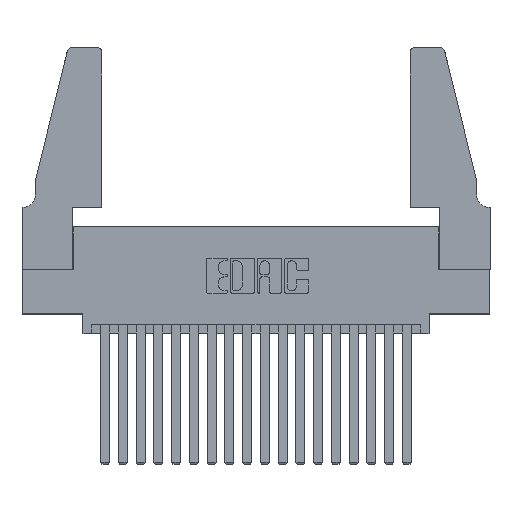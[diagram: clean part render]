
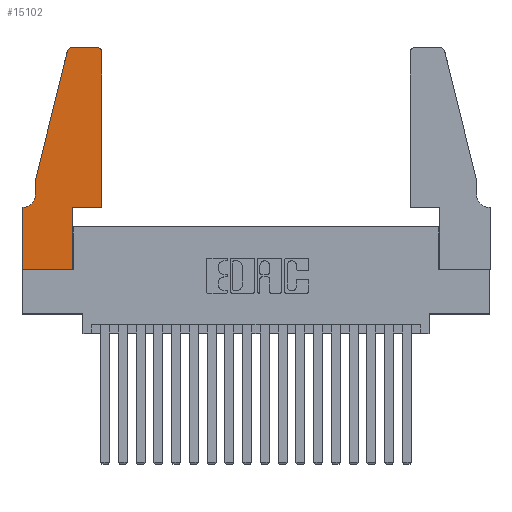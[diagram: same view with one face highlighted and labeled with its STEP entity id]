
A CAD part, top view. The second image highlights one B-rep face of the part: STEP entity #15102.
In plain terms, the highlighted planar face has unit normal (0, 0, 1).
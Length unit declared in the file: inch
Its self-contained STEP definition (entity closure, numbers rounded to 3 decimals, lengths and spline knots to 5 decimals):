
#88 = DIRECTION ( 'NONE',  ( 1., 0., 0. ) ) ;
#147 = DIRECTION ( 'NONE',  ( 0., 1., 0. ) ) ;
#178 = LINE ( 'NONE', #14275, #7966 ) ;
#248 = CARTESIAN_POINT ( 'NONE',  ( 0., 0.35, 0.37 ) ) ;
#522 = ORIENTED_EDGE ( 'NONE', *, *, #8987, .T. ) ;
#708 = CARTESIAN_POINT ( 'NONE',  ( 0.0755, 0.35, 0.37 ) ) ;
#824 = CARTESIAN_POINT ( 'NONE',  ( 0.2865, 0., 0.37 ) ) ;
#938 = VECTOR ( 'NONE', #147, 39.37008 ) ;
#967 = EDGE_LOOP ( 'NONE', ( #17690, #7799, #4221, #8732, #2994, #7582, #4954, #1731, #14276, #15666, #522, #7607 ) ) ;
#1402 = LINE ( 'NONE', #3292, #938 ) ;
#1456 = EDGE_CURVE ( 'NONE', #5873, #14737, #15552, .T. ) ;
#1731 = ORIENTED_EDGE ( 'NONE', *, *, #8331, .T. ) ;
#1837 = PLANE ( 'NONE',  #11635 ) ;
#2092 = VECTOR ( 'NONE', #7995, 39.37008 ) ;
#2198 = CARTESIAN_POINT ( 'NONE',  ( 0.4505, 0.35, 0.37 ) ) ;
#2199 = VERTEX_POINT ( 'NONE', #11678 ) ;
#2308 = VERTEX_POINT ( 'NONE', #9974 ) ;
#2362 = DIRECTION ( 'NONE',  ( 0., 1., 0. ) ) ;
#2425 = EDGE_CURVE ( 'NONE', #12426, #5873, #17566, .T. ) ;
#2835 = AXIS2_PLACEMENT_3D ( 'NONE', #18126, #9344, #88 ) ;
#2994 = ORIENTED_EDGE ( 'NONE', *, *, #18997, .T. ) ;
#3292 = CARTESIAN_POINT ( 'NONE',  ( 0.2865, 0.35, 0.37 ) ) ;
#3478 = DIRECTION ( 'NONE',  ( 0., 0., 1. ) ) ;
#3642 = VECTOR ( 'NONE', #13840, 39.37008 ) ;
#3739 = AXIS2_PLACEMENT_3D ( 'NONE', #7077, #17346, #8544 ) ;
#3792 = LINE ( 'NONE', #2198, #14749 ) ;
#3895 = DIRECTION ( 'NONE',  ( -1., 0., 0. ) ) ;
#3970 = CARTESIAN_POINT ( 'NONE',  ( 0., 0., 0.37 ) ) ;
#4125 = CARTESIAN_POINT ( 'NONE',  ( 0.25487, 1.22718, 0.37 ) ) ;
#4221 = ORIENTED_EDGE ( 'NONE', *, *, #2425, .T. ) ;
#4752 = VERTEX_POINT ( 'NONE', #10241 ) ;
#4954 = ORIENTED_EDGE ( 'NONE', *, *, #5242, .T. ) ;
#5242 = EDGE_CURVE ( 'NONE', #16561, #13067, #178, .T. ) ;
#5262 = EDGE_CURVE ( 'NONE', #18013, #16561, #15336, .T. ) ;
#5575 = CIRCLE ( 'NONE', #3739, 0.03 ) ;
#5873 = VERTEX_POINT ( 'NONE', #11477 ) ;
#5892 = VERTEX_POINT ( 'NONE', #824 ) ;
#6156 = EDGE_CURVE ( 'NONE', #5892, #2308, #1402, .T. ) ;
#6616 = CARTESIAN_POINT ( 'NONE',  ( 0.0055, 0.42, 0.37 ) ) ;
#7077 = CARTESIAN_POINT ( 'NONE',  ( 0.284, 1.22, 0.37 ) ) ;
#7582 = ORIENTED_EDGE ( 'NONE', *, *, #5262, .T. ) ;
#7607 = ORIENTED_EDGE ( 'NONE', *, *, #18281, .T. ) ;
#7799 = ORIENTED_EDGE ( 'NONE', *, *, #16663, .T. ) ;
#7966 = VECTOR ( 'NONE', #8418, 39.37008 ) ;
#7995 = DIRECTION ( 'NONE',  ( -0.239, -0.971, 0. ) ) ;
#8025 = CARTESIAN_POINT ( 'NONE',  ( 0.0755, 0.5, 0.37 ) ) ;
#8038 = CIRCLE ( 'NONE', #18081, 0.07 ) ;
#8085 = DIRECTION ( 'NONE',  ( -1., 0., 0. ) ) ;
#8144 = CARTESIAN_POINT ( 'NONE',  ( 0.2605, 1.25, 0.37 ) ) ;
#8243 = CARTESIAN_POINT ( 'NONE',  ( 0.284, 1.25, 0.37 ) ) ;
#8331 = EDGE_CURVE ( 'NONE', #13067, #5892, #10869, .T. ) ;
#8418 = DIRECTION ( 'NONE',  ( 0., -1., 0. ) ) ;
#8433 = VECTOR ( 'NONE', #15491, 39.37008 ) ;
#8544 = DIRECTION ( 'NONE',  ( 1., 0., 0. ) ) ;
#8732 = ORIENTED_EDGE ( 'NONE', *, *, #1456, .T. ) ;
#8987 = EDGE_CURVE ( 'NONE', #2199, #17456, #14071, .T. ) ;
#9344 = DIRECTION ( 'NONE',  ( 0., 0., 1. ) ) ;
#9970 = VECTOR ( 'NONE', #16020, 39.37008 ) ;
#9974 = CARTESIAN_POINT ( 'NONE',  ( 0.2865, 0.35, 0.37 ) ) ;
#10241 = CARTESIAN_POINT ( 'NONE',  ( 0.4205, 1.25, 0.37 ) ) ;
#10869 = LINE ( 'NONE', #14541, #9970 ) ;
#11420 = VECTOR ( 'NONE', #3895, 39.37008 ) ;
#11477 = CARTESIAN_POINT ( 'NONE',  ( 0.0755, 0.5, 0.37 ) ) ;
#11635 = AXIS2_PLACEMENT_3D ( 'NONE', #248, #3478, #13922 ) ;
#11678 = CARTESIAN_POINT ( 'NONE',  ( 0.4505, 0.35, 0.37 ) ) ;
#11696 = LINE ( 'NONE', #8144, #8433 ) ;
#11744 = CIRCLE ( 'NONE', #2835, 0.03 ) ;
#11911 = FACE_OUTER_BOUND ( 'NONE', #967, .T. ) ;
#12426 = VERTEX_POINT ( 'NONE', #4125 ) ;
#13067 = VERTEX_POINT ( 'NONE', #3970 ) ;
#13660 = EDGE_CURVE ( 'NONE', #2308, #2199, #3792, .T. ) ;
#13840 = DIRECTION ( 'NONE',  ( 0., -1., 0. ) ) ;
#13922 = DIRECTION ( 'NONE',  ( 1., 0., 0. ) ) ;
#14071 = LINE ( 'NONE', #18752, #18436 ) ;
#14138 = CARTESIAN_POINT ( 'NONE',  ( 0., 0.35, 0.37 ) ) ;
#14248 = DIRECTION ( 'NONE',  ( 1., 0., 0. ) ) ;
#14276 = ORIENTED_EDGE ( 'NONE', *, *, #6156, .T. ) ;
#14275 = CARTESIAN_POINT ( 'NONE',  ( 0., 0., 0.37 ) ) ;
#14297 = VERTEX_POINT ( 'NONE', #8243 ) ;
#14532 = CARTESIAN_POINT ( 'NONE',  ( 0.0755, 0.5, 0.37 ) ) ;
#14541 = CARTESIAN_POINT ( 'NONE',  ( 0., 0., 0.37 ) ) ;
#14737 = VERTEX_POINT ( 'NONE', #15166 ) ;
#14749 = VECTOR ( 'NONE', #14248, 39.37008 ) ;
#14910 = EDGE_CURVE ( 'NONE', #4752, #14297, #11696, .T. ) ;
#15102 = ADVANCED_FACE ( 'NONE', ( #11911 ), #1837, .T. ) ;
#15166 = CARTESIAN_POINT ( 'NONE',  ( 0.0755, 0.42, 0.37 ) ) ;
#15336 = LINE ( 'NONE', #708, #11420 ) ;
#15491 = DIRECTION ( 'NONE',  ( -1., 0., 0. ) ) ;
#15552 = LINE ( 'NONE', #14532, #3642 ) ;
#15666 = ORIENTED_EDGE ( 'NONE', *, *, #13660, .T. ) ;
#16020 = DIRECTION ( 'NONE',  ( 1., 0., 0. ) ) ;
#16561 = VERTEX_POINT ( 'NONE', #14138 ) ;
#16663 = EDGE_CURVE ( 'NONE', #14297, #12426, #5575, .T. ) ;
#16897 = DIRECTION ( 'NONE',  ( 0., 0., -1. ) ) ;
#17346 = DIRECTION ( 'NONE',  ( 0., 0., 1. ) ) ;
#17456 = VERTEX_POINT ( 'NONE', #19361 ) ;
#17515 = CARTESIAN_POINT ( 'NONE',  ( 0.0055, 0.35, 0.37 ) ) ;
#17566 = LINE ( 'NONE', #8025, #2092 ) ;
#17690 = ORIENTED_EDGE ( 'NONE', *, *, #14910, .T. ) ;
#18013 = VERTEX_POINT ( 'NONE', #17515 ) ;
#18081 = AXIS2_PLACEMENT_3D ( 'NONE', #6616, #16897, #8085 ) ;
#18126 = CARTESIAN_POINT ( 'NONE',  ( 0.4205, 1.22, 0.37 ) ) ;
#18281 = EDGE_CURVE ( 'NONE', #17456, #4752, #11744, .T. ) ;
#18436 = VECTOR ( 'NONE', #2362, 39.37008 ) ;
#18752 = CARTESIAN_POINT ( 'NONE',  ( 0.4505, 0.35, 0.37 ) ) ;
#18997 = EDGE_CURVE ( 'NONE', #14737, #18013, #8038, .T. ) ;
#19361 = CARTESIAN_POINT ( 'NONE',  ( 0.4505, 1.22, 0.37 ) ) ;
